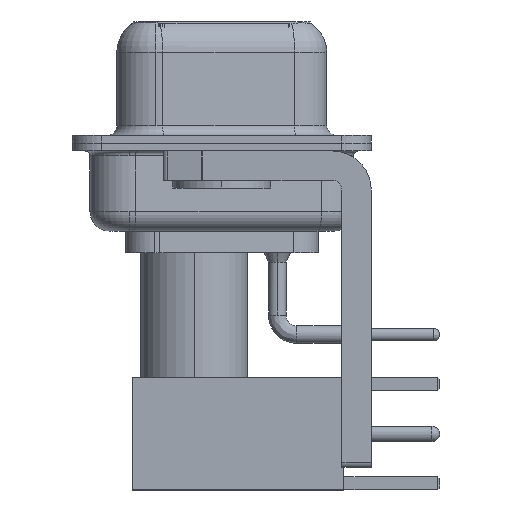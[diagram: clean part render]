
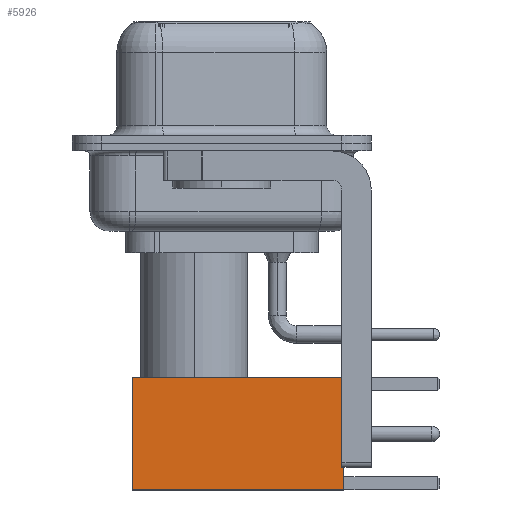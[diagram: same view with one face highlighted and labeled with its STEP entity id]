
A CAD part, left-side view. The second image highlights one B-rep face of the part: STEP entity #5926.
In plain terms, the highlighted face is planar.
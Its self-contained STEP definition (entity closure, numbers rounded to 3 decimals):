
#181 = LINE ( 'NONE', #16600, #11303 ) ;
#727 = VECTOR ( 'NONE', #16589, 1000. ) ;
#1713 = PLANE ( 'NONE',  #6239 ) ;
#1940 = VERTEX_POINT ( 'NONE', #24353 ) ;
#2078 = LINE ( 'NONE', #2206, #727 ) ;
#2206 = CARTESIAN_POINT ( 'NONE',  ( -2.875, 2.875, 0. ) ) ;
#2769 = VECTOR ( 'NONE', #13900, 1000. ) ;
#5926 = ADVANCED_FACE ( 'NONE', ( #13805 ), #1713, .T. ) ;
#6020 = DIRECTION ( 'NONE',  ( -1., 0., 0. ) ) ;
#6239 = AXIS2_PLACEMENT_3D ( 'NONE', #26260, #11621, #17594 ) ;
#7080 = ORIENTED_EDGE ( 'NONE', *, *, #8789, .T. ) ;
#7760 = CARTESIAN_POINT ( 'NONE',  ( 0., 2.875, 10.82 ) ) ;
#8789 = EDGE_CURVE ( 'NONE', #17261, #1940, #13628, .T. ) ;
#11303 = VECTOR ( 'NONE', #6020, 1000. ) ;
#11621 = DIRECTION ( 'NONE',  ( 0., 1., 0. ) ) ;
#11754 = ORIENTED_EDGE ( 'NONE', *, *, #18931, .F. ) ;
#12077 = EDGE_CURVE ( 'NONE', #25667, #24031, #2078, .T. ) ;
#13628 = LINE ( 'NONE', #22169, #2769 ) ;
#13805 = FACE_OUTER_BOUND ( 'NONE', #16133, .T. ) ;
#13900 = DIRECTION ( 'NONE',  ( 0., 0., -1. ) ) ;
#14833 = VECTOR ( 'NONE', #24323, 1000. ) ;
#14913 = CARTESIAN_POINT ( 'NONE',  ( -2.875, 2.875, 0. ) ) ;
#16133 = EDGE_LOOP ( 'NONE', ( #7080, #19070, #20600, #11754 ) ) ;
#16589 = DIRECTION ( 'NONE',  ( 0., 0., -1. ) ) ;
#16600 = CARTESIAN_POINT ( 'NONE',  ( 0., 2.875, 0. ) ) ;
#17261 = VERTEX_POINT ( 'NONE', #23650 ) ;
#17594 = DIRECTION ( 'NONE',  ( 0., 0., 1. ) ) ;
#18931 = EDGE_CURVE ( 'NONE', #17261, #25667, #26346, .T. ) ;
#19070 = ORIENTED_EDGE ( 'NONE', *, *, #19938, .T. ) ;
#19661 = CARTESIAN_POINT ( 'NONE',  ( -2.875, 2.875, 10.82 ) ) ;
#19938 = EDGE_CURVE ( 'NONE', #1940, #24031, #181, .T. ) ;
#20600 = ORIENTED_EDGE ( 'NONE', *, *, #12077, .F. ) ;
#22169 = CARTESIAN_POINT ( 'NONE',  ( 2.875, 2.875, 0. ) ) ;
#23650 = CARTESIAN_POINT ( 'NONE',  ( 2.875, 2.875, 10.82 ) ) ;
#24031 = VERTEX_POINT ( 'NONE', #14913 ) ;
#24323 = DIRECTION ( 'NONE',  ( -1., 0., 0. ) ) ;
#24353 = CARTESIAN_POINT ( 'NONE',  ( 2.875, 2.875, 0. ) ) ;
#25667 = VERTEX_POINT ( 'NONE', #19661 ) ;
#26260 = CARTESIAN_POINT ( 'NONE',  ( 2.875, 2.875, 0. ) ) ;
#26346 = LINE ( 'NONE', #7760, #14833 ) ;
